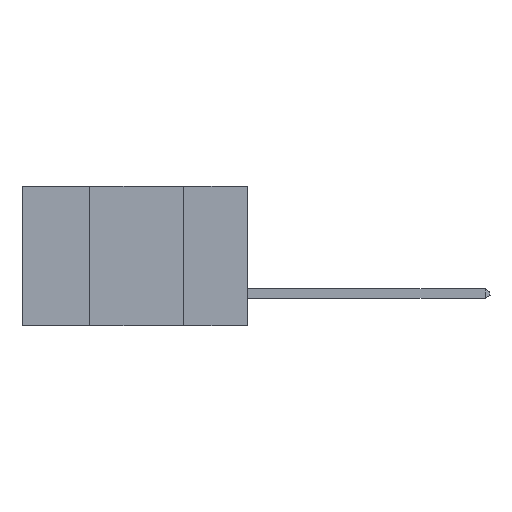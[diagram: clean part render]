
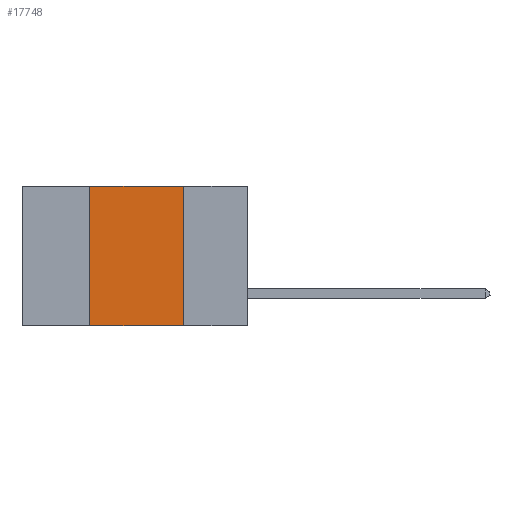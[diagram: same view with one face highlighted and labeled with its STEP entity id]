
A CAD part, left-side view. The second image highlights one B-rep face of the part: STEP entity #17748.
In plain terms, the highlighted planar face has unit normal (-1, 0, 0).
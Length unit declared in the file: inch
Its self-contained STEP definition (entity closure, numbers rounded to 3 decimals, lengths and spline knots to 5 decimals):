
#1502 = VERTEX_POINT ( 'NONE', #6511 ) ;
#2521 = PLANE ( 'NONE',  #4944 ) ;
#4179 = ORIENTED_EDGE ( 'NONE', *, *, #25901, .F. ) ;
#4311 = DIRECTION ( 'NONE',  ( 0., 0., 1. ) ) ;
#4944 = AXIS2_PLACEMENT_3D ( 'NONE', #21139, #14203, #20945 ) ;
#6339 = EDGE_LOOP ( 'NONE', ( #4179, #18879, #7388, #9112 ) ) ;
#6511 = CARTESIAN_POINT ( 'NONE',  ( 0., 0.42, -0.37 ) ) ;
#6694 = CARTESIAN_POINT ( 'NONE',  ( 0., 0.17, 0. ) ) ;
#7388 = ORIENTED_EDGE ( 'NONE', *, *, #12050, .F. ) ;
#7801 = LINE ( 'NONE', #27138, #15784 ) ;
#7937 = FACE_OUTER_BOUND ( 'NONE', #6339, .T. ) ;
#8187 = VERTEX_POINT ( 'NONE', #6694 ) ;
#8915 = CARTESIAN_POINT ( 'NONE',  ( 0., 0.6, 0. ) ) ;
#8928 = DIRECTION ( 'NONE',  ( 0., -1., 0. ) ) ;
#9048 = CARTESIAN_POINT ( 'NONE',  ( 0., 0.42, 0. ) ) ;
#9112 = ORIENTED_EDGE ( 'NONE', *, *, #10107, .T. ) ;
#10064 = VECTOR ( 'NONE', #23714, 39.37008 ) ;
#10107 = EDGE_CURVE ( 'NONE', #1502, #24329, #18122, .T. ) ;
#10937 = DIRECTION ( 'NONE',  ( 0., 0., -1. ) ) ;
#12050 = EDGE_CURVE ( 'NONE', #1502, #17286, #20209, .T. ) ;
#14004 = VECTOR ( 'NONE', #4311, 39.37008 ) ;
#14203 = DIRECTION ( 'NONE',  ( 1., 0., 0. ) ) ;
#15784 = VECTOR ( 'NONE', #10937, 39.37008 ) ;
#17286 = VERTEX_POINT ( 'NONE', #29274 ) ;
#17748 = ADVANCED_FACE ( 'NONE', ( #7937 ), #2521, .F. ) ;
#18065 = CARTESIAN_POINT ( 'NONE',  ( 0., 0.6, -0.37 ) ) ;
#18122 = LINE ( 'NONE', #18065, #18874 ) ;
#18874 = VECTOR ( 'NONE', #8928, 39.37008 ) ;
#18879 = ORIENTED_EDGE ( 'NONE', *, *, #23395, .F. ) ;
#20209 = LINE ( 'NONE', #9048, #14004 ) ;
#20945 = DIRECTION ( 'NONE',  ( 0., 0., -1. ) ) ;
#21035 = LINE ( 'NONE', #8915, #10064 ) ;
#21139 = CARTESIAN_POINT ( 'NONE',  ( 0., 0.6, 0. ) ) ;
#23395 = EDGE_CURVE ( 'NONE', #17286, #8187, #21035, .T. ) ;
#23714 = DIRECTION ( 'NONE',  ( 0., -1., 0. ) ) ;
#24329 = VERTEX_POINT ( 'NONE', #29831 ) ;
#25901 = EDGE_CURVE ( 'NONE', #8187, #24329, #7801, .T. ) ;
#27138 = CARTESIAN_POINT ( 'NONE',  ( 0., 0.17, 0. ) ) ;
#29274 = CARTESIAN_POINT ( 'NONE',  ( 0., 0.42, 0. ) ) ;
#29831 = CARTESIAN_POINT ( 'NONE',  ( 0., 0.17, -0.37 ) ) ;
